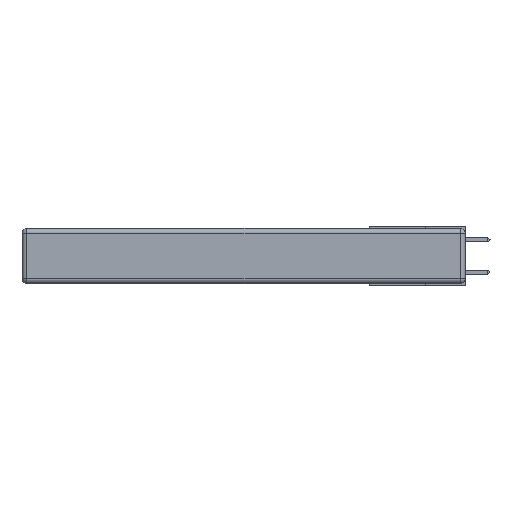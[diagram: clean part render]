
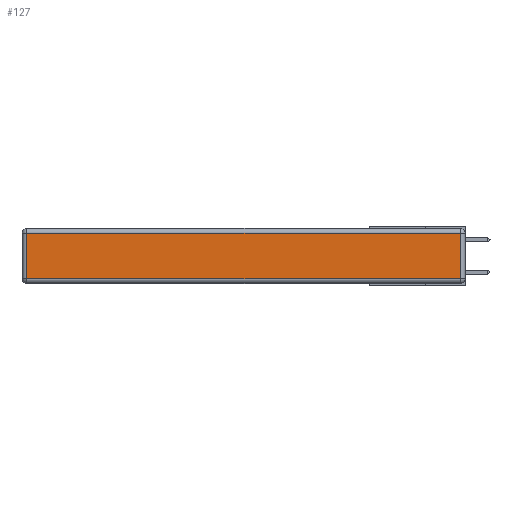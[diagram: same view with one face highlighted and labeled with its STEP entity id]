
A CAD part, left-side view. The second image highlights one B-rep face of the part: STEP entity #127.
In plain terms, the highlighted planar face has unit normal (-1, 0, 0).
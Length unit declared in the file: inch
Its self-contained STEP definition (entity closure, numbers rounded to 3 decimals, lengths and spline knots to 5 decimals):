
#45 = EDGE_CURVE ( 'NONE', #13882, #2330, #4500, .T. ) ;
#66 = CARTESIAN_POINT ( 'NONE',  ( 0., 0.03, -0.343 ) ) ;
#127 = ADVANCED_FACE ( 'NONE', ( #5393 ), #11923, .T. ) ;
#832 = CARTESIAN_POINT ( 'NONE',  ( 0., 0.03, -0.313 ) ) ;
#1097 = LINE ( 'NONE', #66, #11724 ) ;
#1105 = VECTOR ( 'NONE', #4047, 39.37008 ) ;
#1129 = DIRECTION ( 'NONE',  ( 0., 0., 1. ) ) ;
#1810 = CARTESIAN_POINT ( 'NONE',  ( 0., 0., -0.343 ) ) ;
#2079 = CARTESIAN_POINT ( 'NONE',  ( 0., 2.72, -0.313 ) ) ;
#2330 = VERTEX_POINT ( 'NONE', #2079 ) ;
#2904 = CARTESIAN_POINT ( 'NONE',  ( 0., 2.75, -0.03 ) ) ;
#2941 = DIRECTION ( 'NONE',  ( 0., 0., -1. ) ) ;
#3333 = ORIENTED_EDGE ( 'NONE', *, *, #6435, .T. ) ;
#3672 = CARTESIAN_POINT ( 'NONE',  ( 0., 2.72, -0.03 ) ) ;
#3725 = DIRECTION ( 'NONE',  ( 0., -1., 0. ) ) ;
#3789 = VECTOR ( 'NONE', #3725, 39.37008 ) ;
#4047 = DIRECTION ( 'NONE',  ( 0., 1., 0. ) ) ;
#4500 = LINE ( 'NONE', #7283, #5026 ) ;
#5026 = VECTOR ( 'NONE', #2941, 39.37008 ) ;
#5125 = DIRECTION ( 'NONE',  ( -1., 0., 0. ) ) ;
#5128 = VERTEX_POINT ( 'NONE', #832 ) ;
#5274 = VERTEX_POINT ( 'NONE', #8884 ) ;
#5367 = ORIENTED_EDGE ( 'NONE', *, *, #9339, .T. ) ;
#5393 = FACE_OUTER_BOUND ( 'NONE', #13824, .T. ) ;
#6042 = ORIENTED_EDGE ( 'NONE', *, *, #45, .T. ) ;
#6108 = CARTESIAN_POINT ( 'NONE',  ( 0., 0., -0.313 ) ) ;
#6435 = EDGE_CURVE ( 'NONE', #2330, #5128, #7292, .T. ) ;
#7283 = CARTESIAN_POINT ( 'NONE',  ( 0., 2.72, -0.343 ) ) ;
#7292 = LINE ( 'NONE', #6108, #3789 ) ;
#8694 = AXIS2_PLACEMENT_3D ( 'NONE', #1810, #5125, #9687 ) ;
#8884 = CARTESIAN_POINT ( 'NONE',  ( 0., 0.03, -0.03 ) ) ;
#9339 = EDGE_CURVE ( 'NONE', #5274, #13882, #10468, .T. ) ;
#9687 = DIRECTION ( 'NONE',  ( 0., 0., 1. ) ) ;
#10468 = LINE ( 'NONE', #2904, #1105 ) ;
#10690 = EDGE_CURVE ( 'NONE', #5128, #5274, #1097, .T. ) ;
#11724 = VECTOR ( 'NONE', #1129, 39.37008 ) ;
#11923 = PLANE ( 'NONE',  #8694 ) ;
#12192 = ORIENTED_EDGE ( 'NONE', *, *, #10690, .T. ) ;
#13824 = EDGE_LOOP ( 'NONE', ( #3333, #12192, #5367, #6042 ) ) ;
#13882 = VERTEX_POINT ( 'NONE', #3672 ) ;
